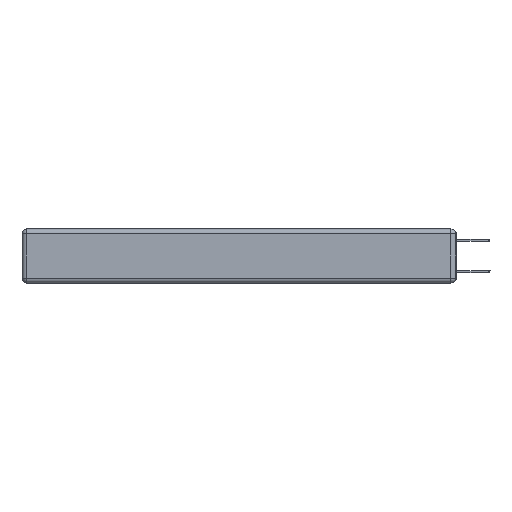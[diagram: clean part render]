
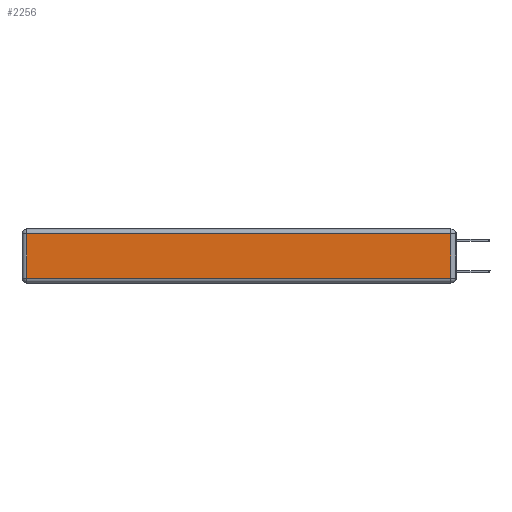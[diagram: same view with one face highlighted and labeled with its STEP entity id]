
A CAD part, left-side view. The second image highlights one B-rep face of the part: STEP entity #2256.
In plain terms, the highlighted planar face has unit normal (-1, 0, 0).
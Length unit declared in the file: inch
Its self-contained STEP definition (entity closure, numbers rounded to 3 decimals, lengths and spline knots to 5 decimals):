
#18 = CARTESIAN_POINT ( 'NONE',  ( 0., 0.03, -0.03 ) ) ;
#525 = CARTESIAN_POINT ( 'NONE',  ( 0., 0., -0.313 ) ) ;
#532 = CARTESIAN_POINT ( 'NONE',  ( 0., 2.72, -0.313 ) ) ;
#1441 = CARTESIAN_POINT ( 'NONE',  ( 0., 2.75, -0.03 ) ) ;
#1477 = EDGE_CURVE ( 'NONE', #5508, #4857, #2662, .T. ) ;
#2256 = ADVANCED_FACE ( 'NONE', ( #16715 ), #16979, .T. ) ;
#2662 = LINE ( 'NONE', #10192, #10659 ) ;
#3756 = LINE ( 'NONE', #13671, #10024 ) ;
#4217 = DIRECTION ( 'NONE',  ( -1., 0., 0. ) ) ;
#4226 = CARTESIAN_POINT ( 'NONE',  ( 0., 2.72, -0.03 ) ) ;
#4857 = VERTEX_POINT ( 'NONE', #532 ) ;
#4881 = AXIS2_PLACEMENT_3D ( 'NONE', #6049, #4217, #11463 ) ;
#5127 = CARTESIAN_POINT ( 'NONE',  ( 0., 0.03, -0.313 ) ) ;
#5508 = VERTEX_POINT ( 'NONE', #4226 ) ;
#5874 = ORIENTED_EDGE ( 'NONE', *, *, #6270, .T. ) ;
#6049 = CARTESIAN_POINT ( 'NONE',  ( 0., 0., -0.343 ) ) ;
#6250 = DIRECTION ( 'NONE',  ( 0., -1., 0. ) ) ;
#6270 = EDGE_CURVE ( 'NONE', #17219, #5508, #16662, .T. ) ;
#6832 = DIRECTION ( 'NONE',  ( 0., 0., 1. ) ) ;
#8313 = VECTOR ( 'NONE', #6250, 39.37008 ) ;
#10024 = VECTOR ( 'NONE', #6832, 39.37008 ) ;
#10192 = CARTESIAN_POINT ( 'NONE',  ( 0., 2.72, -0.343 ) ) ;
#10267 = LINE ( 'NONE', #525, #8313 ) ;
#10659 = VECTOR ( 'NONE', #11529, 39.37008 ) ;
#11463 = DIRECTION ( 'NONE',  ( 0., 0., 1. ) ) ;
#11529 = DIRECTION ( 'NONE',  ( 0., 0., -1. ) ) ;
#12807 = EDGE_CURVE ( 'NONE', #4857, #17140, #10267, .T. ) ;
#13132 = EDGE_CURVE ( 'NONE', #17140, #17219, #3756, .T. ) ;
#13671 = CARTESIAN_POINT ( 'NONE',  ( 0., 0.03, -0.343 ) ) ;
#15095 = EDGE_LOOP ( 'NONE', ( #15155, #16524, #5874, #16070 ) ) ;
#15155 = ORIENTED_EDGE ( 'NONE', *, *, #12807, .T. ) ;
#15215 = DIRECTION ( 'NONE',  ( 0., 1., 0. ) ) ;
#16070 = ORIENTED_EDGE ( 'NONE', *, *, #1477, .T. ) ;
#16524 = ORIENTED_EDGE ( 'NONE', *, *, #13132, .T. ) ;
#16662 = LINE ( 'NONE', #1441, #17520 ) ;
#16715 = FACE_OUTER_BOUND ( 'NONE', #15095, .T. ) ;
#16979 = PLANE ( 'NONE',  #4881 ) ;
#17140 = VERTEX_POINT ( 'NONE', #5127 ) ;
#17219 = VERTEX_POINT ( 'NONE', #18 ) ;
#17520 = VECTOR ( 'NONE', #15215, 39.37008 ) ;
